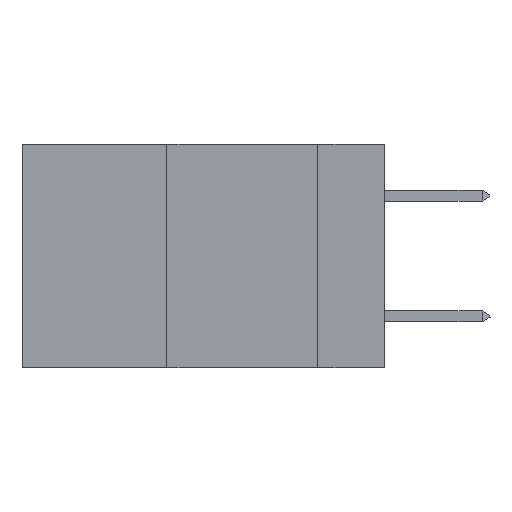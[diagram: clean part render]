
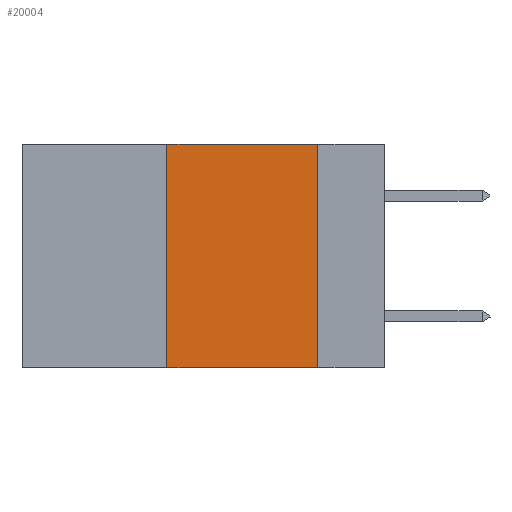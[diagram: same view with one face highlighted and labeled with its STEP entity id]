
A CAD part, left-side view. The second image highlights one B-rep face of the part: STEP entity #20004.
In plain terms, the highlighted planar face has unit normal (-1, 0, 0).
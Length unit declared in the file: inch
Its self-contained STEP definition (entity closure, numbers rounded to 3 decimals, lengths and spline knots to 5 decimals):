
#129 = ORIENTED_EDGE ( 'NONE', *, *, #17028, .T. ) ;
#1205 = VERTEX_POINT ( 'NONE', #11202 ) ;
#2895 = VECTOR ( 'NONE', #19047, 39.37008 ) ;
#3369 = AXIS2_PLACEMENT_3D ( 'NONE', #37991, #18093, #41253 ) ;
#3813 = FACE_OUTER_BOUND ( 'NONE', #7956, .T. ) ;
#5228 = VECTOR ( 'NONE', #12944, 39.37008 ) ;
#7563 = EDGE_CURVE ( 'NONE', #41223, #1205, #12081, .T. ) ;
#7720 = CARTESIAN_POINT ( 'NONE',  ( 0., 0.11, -0.37 ) ) ;
#7956 = EDGE_LOOP ( 'NONE', ( #13542, #28483, #14176, #129 ) ) ;
#8660 = CARTESIAN_POINT ( 'NONE',  ( 0., 0.36, -0.37 ) ) ;
#9621 = CARTESIAN_POINT ( 'NONE',  ( 0., 0.6, -0.37 ) ) ;
#10265 = CARTESIAN_POINT ( 'NONE',  ( 0., 0.36, 0. ) ) ;
#11202 = CARTESIAN_POINT ( 'NONE',  ( 0., 0.11, 0. ) ) ;
#11655 = EDGE_CURVE ( 'NONE', #1205, #13304, #36254, .T. ) ;
#12081 = LINE ( 'NONE', #22188, #2895 ) ;
#12944 = DIRECTION ( 'NONE',  ( 0., -1., 0. ) ) ;
#13304 = VERTEX_POINT ( 'NONE', #7720 ) ;
#13542 = ORIENTED_EDGE ( 'NONE', *, *, #11655, .F. ) ;
#13746 = DIRECTION ( 'NONE',  ( 0., 0., 1. ) ) ;
#14176 = ORIENTED_EDGE ( 'NONE', *, *, #18567, .F. ) ;
#14365 = DIRECTION ( 'NONE',  ( 0., 0., -1. ) ) ;
#14659 = PLANE ( 'NONE',  #3369 ) ;
#17028 = EDGE_CURVE ( 'NONE', #35556, #13304, #38930, .T. ) ;
#17529 = VECTOR ( 'NONE', #14365, 39.37008 ) ;
#18093 = DIRECTION ( 'NONE',  ( 1., 0., 0. ) ) ;
#18567 = EDGE_CURVE ( 'NONE', #35556, #41223, #21183, .T. ) ;
#19047 = DIRECTION ( 'NONE',  ( 0., -1., 0. ) ) ;
#20004 = ADVANCED_FACE ( 'NONE', ( #3813 ), #14659, .F. ) ;
#21183 = LINE ( 'NONE', #10265, #36699 ) ;
#22188 = CARTESIAN_POINT ( 'NONE',  ( 0., 0.6, 0. ) ) ;
#28483 = ORIENTED_EDGE ( 'NONE', *, *, #7563, .F. ) ;
#30131 = CARTESIAN_POINT ( 'NONE',  ( 0., 0.36, 0. ) ) ;
#35556 = VERTEX_POINT ( 'NONE', #8660 ) ;
#36254 = LINE ( 'NONE', #37711, #17529 ) ;
#36699 = VECTOR ( 'NONE', #13746, 39.37008 ) ;
#37711 = CARTESIAN_POINT ( 'NONE',  ( 0., 0.11, 0. ) ) ;
#37991 = CARTESIAN_POINT ( 'NONE',  ( 0., 0.6, 0. ) ) ;
#38930 = LINE ( 'NONE', #9621, #5228 ) ;
#41223 = VERTEX_POINT ( 'NONE', #30131 ) ;
#41253 = DIRECTION ( 'NONE',  ( 0., 0., -1. ) ) ;
